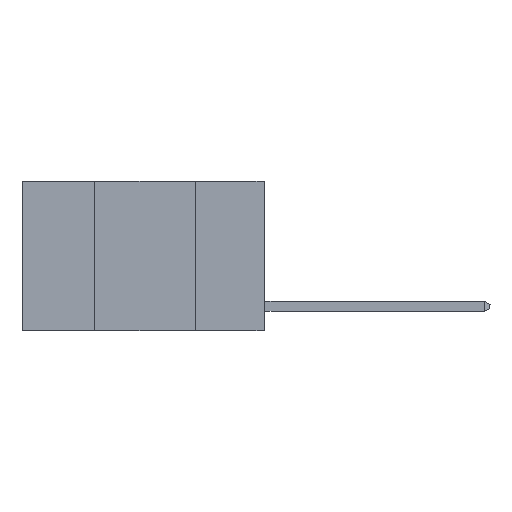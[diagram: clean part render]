
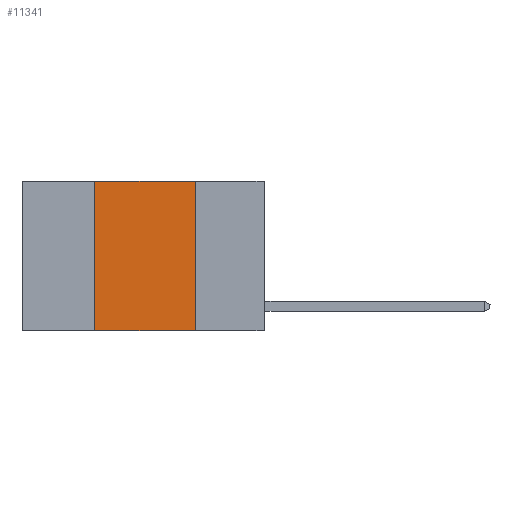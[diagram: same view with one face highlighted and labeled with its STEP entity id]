
A CAD part, left-side view. The second image highlights one B-rep face of the part: STEP entity #11341.
In plain terms, the highlighted planar face has unit normal (-1, 0, 0).
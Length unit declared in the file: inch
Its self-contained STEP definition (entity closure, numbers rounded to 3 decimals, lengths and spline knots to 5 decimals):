
#910 = EDGE_CURVE ( 'NONE', #6624, #4477, #2693, .T. ) ;
#996 = LINE ( 'NONE', #7254, #4046 ) ;
#1629 = DIRECTION ( 'NONE',  ( 0., 0., -1. ) ) ;
#1935 = EDGE_CURVE ( 'NONE', #6624, #5294, #7085, .T. ) ;
#2296 = EDGE_CURVE ( 'NONE', #5294, #16440, #996, .T. ) ;
#2693 = LINE ( 'NONE', #19398, #11612 ) ;
#2839 = DIRECTION ( 'NONE',  ( 1., 0., 0. ) ) ;
#3454 = DIRECTION ( 'NONE',  ( 0., 0., -1. ) ) ;
#4046 = VECTOR ( 'NONE', #6965, 39.37008 ) ;
#4477 = VERTEX_POINT ( 'NONE', #14493 ) ;
#5294 = VERTEX_POINT ( 'NONE', #11739 ) ;
#6624 = VERTEX_POINT ( 'NONE', #13338 ) ;
#6965 = DIRECTION ( 'NONE',  ( 0., -1., 0. ) ) ;
#7024 = ORIENTED_EDGE ( 'NONE', *, *, #9104, .F. ) ;
#7085 = LINE ( 'NONE', #13183, #11684 ) ;
#7254 = CARTESIAN_POINT ( 'NONE',  ( 0., 0.6, 0. ) ) ;
#7476 = CARTESIAN_POINT ( 'NONE',  ( 0., 0.17, 0. ) ) ;
#8664 = VECTOR ( 'NONE', #3454, 39.37008 ) ;
#9101 = ORIENTED_EDGE ( 'NONE', *, *, #1935, .F. ) ;
#9104 = EDGE_CURVE ( 'NONE', #16440, #4477, #10633, .T. ) ;
#9276 = EDGE_LOOP ( 'NONE', ( #7024, #19363, #9101, #14519 ) ) ;
#10633 = LINE ( 'NONE', #15491, #8664 ) ;
#11341 = ADVANCED_FACE ( 'NONE', ( #12292 ), #15263, .F. ) ;
#11612 = VECTOR ( 'NONE', #11651, 39.37008 ) ;
#11651 = DIRECTION ( 'NONE',  ( 0., -1., 0. ) ) ;
#11684 = VECTOR ( 'NONE', #19226, 39.37008 ) ;
#11739 = CARTESIAN_POINT ( 'NONE',  ( 0., 0.42, 0. ) ) ;
#11990 = CARTESIAN_POINT ( 'NONE',  ( 0., 0.6, 0. ) ) ;
#12292 = FACE_OUTER_BOUND ( 'NONE', #9276, .T. ) ;
#13183 = CARTESIAN_POINT ( 'NONE',  ( 0., 0.42, 0. ) ) ;
#13338 = CARTESIAN_POINT ( 'NONE',  ( 0., 0.42, -0.37 ) ) ;
#14396 = AXIS2_PLACEMENT_3D ( 'NONE', #11990, #2839, #1629 ) ;
#14493 = CARTESIAN_POINT ( 'NONE',  ( 0., 0.17, -0.37 ) ) ;
#14519 = ORIENTED_EDGE ( 'NONE', *, *, #910, .T. ) ;
#15263 = PLANE ( 'NONE',  #14396 ) ;
#15491 = CARTESIAN_POINT ( 'NONE',  ( 0., 0.17, 0. ) ) ;
#16440 = VERTEX_POINT ( 'NONE', #7476 ) ;
#19226 = DIRECTION ( 'NONE',  ( 0., 0., 1. ) ) ;
#19363 = ORIENTED_EDGE ( 'NONE', *, *, #2296, .F. ) ;
#19398 = CARTESIAN_POINT ( 'NONE',  ( 0., 0.6, -0.37 ) ) ;
